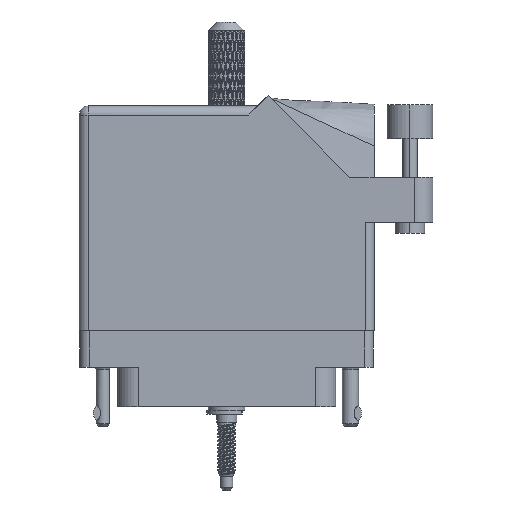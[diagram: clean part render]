
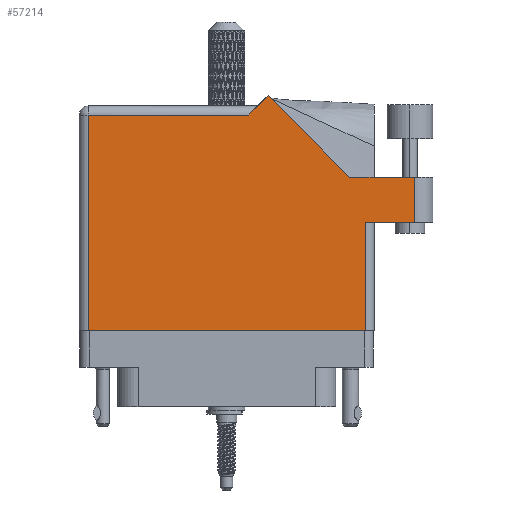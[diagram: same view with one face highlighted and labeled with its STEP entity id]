
A CAD part, front view. The second image highlights one B-rep face of the part: STEP entity #57214.
In plain terms, the highlighted face is planar.
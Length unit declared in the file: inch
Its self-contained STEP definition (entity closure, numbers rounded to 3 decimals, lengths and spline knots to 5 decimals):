
#951 = VECTOR ( 'NONE', #82515, 39.37008 ) ;
#2437 = EDGE_CURVE ( 'NONE', #24549, #43005, #41776, .T. ) ;
#6593 = CARTESIAN_POINT ( 'NONE',  ( -0.943, -0.1, 0.455 ) ) ;
#7581 = DIRECTION ( 'NONE',  ( 0., -1., 0. ) ) ;
#8203 = LINE ( 'NONE', #94490, #65047 ) ;
#8383 = ORIENTED_EDGE ( 'NONE', *, *, #23663, .T. ) ;
#8665 = LINE ( 'NONE', #85560, #86365 ) ;
#9090 = ORIENTED_EDGE ( 'NONE', *, *, #106337, .T. ) ;
#12155 = LINE ( 'NONE', #47212, #951 ) ;
#14069 = EDGE_CURVE ( 'NONE', #64445, #87278, #12155, .T. ) ;
#14417 = EDGE_LOOP ( 'NONE', ( #89824, #9090, #58774, #99264, #113336, #103943, #48225, #8383, #77106 ) ) ;
#15514 = CARTESIAN_POINT ( 'NONE',  ( 0.15, 1.368, 0.455 ) ) ;
#16136 = CARTESIAN_POINT ( 'NONE',  ( -1.005, 1.43, 0.455 ) ) ;
#16610 = CARTESIAN_POINT ( 'NONE',  ( 0.83942, 0.944, 0.455 ) ) ;
#17336 = DIRECTION ( 'NONE',  ( -1., 0., 0. ) ) ;
#21947 = EDGE_CURVE ( 'NONE', #75546, #81803, #89607, .T. ) ;
#22419 = FACE_OUTER_BOUND ( 'NONE', #14417, .T. ) ;
#23499 = DIRECTION ( 'NONE',  ( 1., 0., 0. ) ) ;
#23663 = EDGE_CURVE ( 'NONE', #71926, #24549, #42195, .T. ) ;
#24549 = VERTEX_POINT ( 'NONE', #64527 ) ;
#27999 = EDGE_CURVE ( 'NONE', #102903, #75546, #54906, .T. ) ;
#30072 = CARTESIAN_POINT ( 'NONE',  ( 1.005, 0.637, 0.455 ) ) ;
#31103 = VECTOR ( 'NONE', #68202, 39.37008 ) ;
#32780 = PLANE ( 'NONE',  #100589 ) ;
#33780 = LINE ( 'NONE', #30072, #86579 ) ;
#38979 = VECTOR ( 'NONE', #64976, 39.37008 ) ;
#41776 = LINE ( 'NONE', #66150, #38979 ) ;
#42195 = LINE ( 'NONE', #78590, #83853 ) ;
#43005 = VERTEX_POINT ( 'NONE', #84048 ) ;
#43688 = DIRECTION ( 'NONE',  ( 1., 0., 0. ) ) ;
#45825 = VERTEX_POINT ( 'NONE', #76642 ) ;
#47212 = CARTESIAN_POINT ( 'NONE',  ( -1.005, 1.368, 0.455 ) ) ;
#48225 = ORIENTED_EDGE ( 'NONE', *, *, #77829, .T. ) ;
#51319 = DIRECTION ( 'NONE',  ( -1., 0., 0. ) ) ;
#51800 = DIRECTION ( 'NONE',  ( -0.707, 0.707, 0. ) ) ;
#52114 = VECTOR ( 'NONE', #17336, 39.37008 ) ;
#52558 = EDGE_CURVE ( 'NONE', #81803, #64445, #76982, .T. ) ;
#53044 = EDGE_CURVE ( 'NONE', #43005, #45825, #33780, .T. ) ;
#54906 = LINE ( 'NONE', #97557, #52114 ) ;
#57214 = ADVANCED_FACE ( 'NONE', ( #22419 ), #32780, .F. ) ;
#57748 = CARTESIAN_POINT ( 'NONE',  ( 1.28, 0.944, 0.455 ) ) ;
#58774 = ORIENTED_EDGE ( 'NONE', *, *, #27999, .T. ) ;
#64445 = VERTEX_POINT ( 'NONE', #15514 ) ;
#64527 = CARTESIAN_POINT ( 'NONE',  ( 0.943, -0.1, 0.455 ) ) ;
#64976 = DIRECTION ( 'NONE',  ( 0., 1., 0. ) ) ;
#65047 = VECTOR ( 'NONE', #7581, 39.37008 ) ;
#66150 = CARTESIAN_POINT ( 'NONE',  ( 0.943, 0.637, 0.455 ) ) ;
#68202 = DIRECTION ( 'NONE',  ( -0.707, -0.707, 0. ) ) ;
#71926 = VERTEX_POINT ( 'NONE', #6593 ) ;
#75546 = VERTEX_POINT ( 'NONE', #92092 ) ;
#76642 = CARTESIAN_POINT ( 'NONE',  ( 1.28, 0.637, 0.455 ) ) ;
#76982 = LINE ( 'NONE', #103549, #31103 ) ;
#77106 = ORIENTED_EDGE ( 'NONE', *, *, #2437, .T. ) ;
#77829 = EDGE_CURVE ( 'NONE', #87278, #71926, #8203, .T. ) ;
#78590 = CARTESIAN_POINT ( 'NONE',  ( -1.005, -0.1, 0.455 ) ) ;
#81803 = VERTEX_POINT ( 'NONE', #103166 ) ;
#82515 = DIRECTION ( 'NONE',  ( -1., 0., 0. ) ) ;
#83853 = VECTOR ( 'NONE', #43688, 39.37008 ) ;
#84048 = CARTESIAN_POINT ( 'NONE',  ( 0.943, 0.637, 0.455 ) ) ;
#85560 = CARTESIAN_POINT ( 'NONE',  ( 1.28, 0.944, 0.455 ) ) ;
#86365 = VECTOR ( 'NONE', #102637, 39.37008 ) ;
#86579 = VECTOR ( 'NONE', #23499, 39.37008 ) ;
#87278 = VERTEX_POINT ( 'NONE', #106941 ) ;
#89607 = LINE ( 'NONE', #16610, #107697 ) ;
#89824 = ORIENTED_EDGE ( 'NONE', *, *, #53044, .T. ) ;
#92092 = CARTESIAN_POINT ( 'NONE',  ( 0.83942, 0.944, 0.455 ) ) ;
#94490 = CARTESIAN_POINT ( 'NONE',  ( -0.943, -0.1, 0.455 ) ) ;
#97557 = CARTESIAN_POINT ( 'NONE',  ( 1.405, 0.944, 0.455 ) ) ;
#99264 = ORIENTED_EDGE ( 'NONE', *, *, #21947, .T. ) ;
#100589 = AXIS2_PLACEMENT_3D ( 'NONE', #16136, #112700, #51319 ) ;
#102637 = DIRECTION ( 'NONE',  ( 0., 1., 0. ) ) ;
#102903 = VERTEX_POINT ( 'NONE', #57748 ) ;
#103166 = CARTESIAN_POINT ( 'NONE',  ( 0.28271, 1.50071, 0.455 ) ) ;
#103549 = CARTESIAN_POINT ( 'NONE',  ( 0.212, 1.43, 0.455 ) ) ;
#103943 = ORIENTED_EDGE ( 'NONE', *, *, #14069, .T. ) ;
#106337 = EDGE_CURVE ( 'NONE', #45825, #102903, #8665, .T. ) ;
#106941 = CARTESIAN_POINT ( 'NONE',  ( -0.943, 1.368, 0.455 ) ) ;
#107697 = VECTOR ( 'NONE', #51800, 39.37008 ) ;
#112700 = DIRECTION ( 'NONE',  ( 0., 0., -1. ) ) ;
#113336 = ORIENTED_EDGE ( 'NONE', *, *, #52558, .T. ) ;
